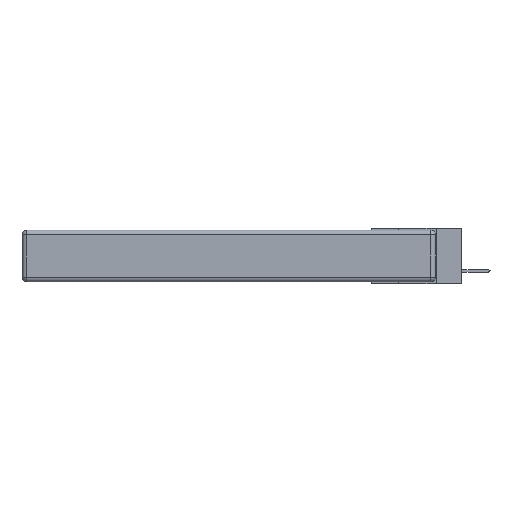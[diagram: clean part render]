
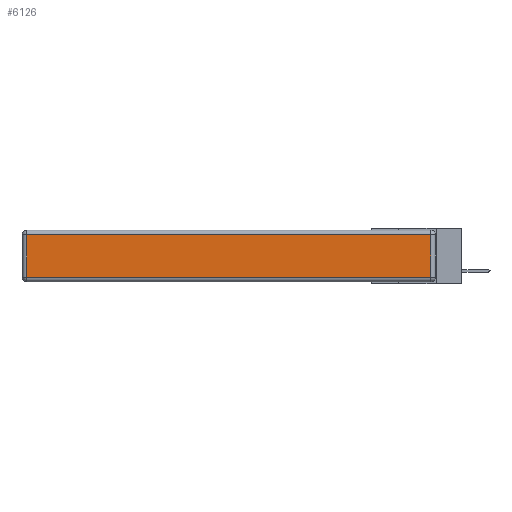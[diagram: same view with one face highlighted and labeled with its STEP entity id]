
A CAD part, left-side view. The second image highlights one B-rep face of the part: STEP entity #6126.
In plain terms, the highlighted planar face has unit normal (-1, 0, 0).
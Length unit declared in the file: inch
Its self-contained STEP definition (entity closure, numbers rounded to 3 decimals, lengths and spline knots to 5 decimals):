
#228 = PLANE ( 'NONE',  #1196 ) ;
#398 = VECTOR ( 'NONE', #4877, 39.37008 ) ;
#483 = FACE_OUTER_BOUND ( 'NONE', #1483, .T. ) ;
#810 = CARTESIAN_POINT ( 'NONE',  ( 0., 2.72, -0.03 ) ) ;
#934 = VERTEX_POINT ( 'NONE', #810 ) ;
#1168 = DIRECTION ( 'NONE',  ( 0., 0., 1. ) ) ;
#1196 = AXIS2_PLACEMENT_3D ( 'NONE', #7152, #1215, #1168 ) ;
#1215 = DIRECTION ( 'NONE',  ( -1., 0., 0. ) ) ;
#1246 = CARTESIAN_POINT ( 'NONE',  ( 0., 2.72, -0.313 ) ) ;
#1483 = EDGE_LOOP ( 'NONE', ( #6986, #5999, #2878, #9737 ) ) ;
#2372 = EDGE_CURVE ( 'NONE', #11113, #12750, #7013, .T. ) ;
#2519 = VECTOR ( 'NONE', #10784, 39.37008 ) ;
#2682 = EDGE_CURVE ( 'NONE', #12750, #5605, #8268, .T. ) ;
#2878 = ORIENTED_EDGE ( 'NONE', *, *, #8830, .T. ) ;
#3818 = CARTESIAN_POINT ( 'NONE',  ( 0., 2.75, -0.03 ) ) ;
#3936 = CARTESIAN_POINT ( 'NONE',  ( 0., 2.72, -0.343 ) ) ;
#4353 = CARTESIAN_POINT ( 'NONE',  ( 0., 0.03, -0.313 ) ) ;
#4562 = CARTESIAN_POINT ( 'NONE',  ( 0., 0., -0.313 ) ) ;
#4877 = DIRECTION ( 'NONE',  ( 0., 1., 0. ) ) ;
#5497 = DIRECTION ( 'NONE',  ( 0., 0., 1. ) ) ;
#5605 = VERTEX_POINT ( 'NONE', #11723 ) ;
#5999 = ORIENTED_EDGE ( 'NONE', *, *, #2682, .T. ) ;
#6126 = ADVANCED_FACE ( 'NONE', ( #483 ), #228, .T. ) ;
#6535 = VECTOR ( 'NONE', #5497, 39.37008 ) ;
#6625 = CARTESIAN_POINT ( 'NONE',  ( 0., 0.03, -0.343 ) ) ;
#6922 = LINE ( 'NONE', #3818, #398 ) ;
#6986 = ORIENTED_EDGE ( 'NONE', *, *, #2372, .T. ) ;
#7013 = LINE ( 'NONE', #4562, #12203 ) ;
#7152 = CARTESIAN_POINT ( 'NONE',  ( 0., 0., -0.343 ) ) ;
#8268 = LINE ( 'NONE', #6625, #6535 ) ;
#8830 = EDGE_CURVE ( 'NONE', #5605, #934, #6922, .T. ) ;
#9737 = ORIENTED_EDGE ( 'NONE', *, *, #12748, .T. ) ;
#10414 = LINE ( 'NONE', #3936, #2519 ) ;
#10784 = DIRECTION ( 'NONE',  ( 0., 0., -1. ) ) ;
#11113 = VERTEX_POINT ( 'NONE', #1246 ) ;
#11391 = DIRECTION ( 'NONE',  ( 0., -1., 0. ) ) ;
#11723 = CARTESIAN_POINT ( 'NONE',  ( 0., 0.03, -0.03 ) ) ;
#12203 = VECTOR ( 'NONE', #11391, 39.37008 ) ;
#12748 = EDGE_CURVE ( 'NONE', #934, #11113, #10414, .T. ) ;
#12750 = VERTEX_POINT ( 'NONE', #4353 ) ;
